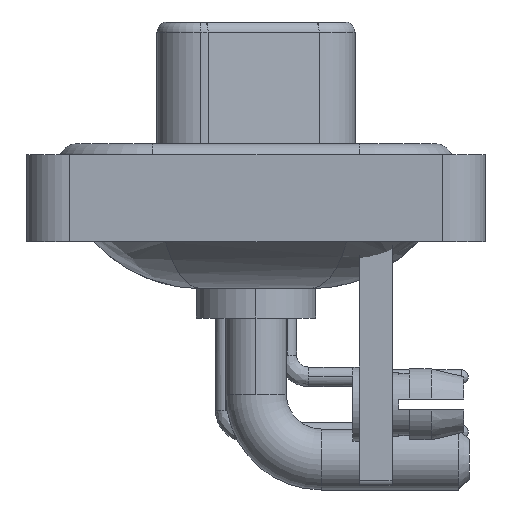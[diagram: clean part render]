
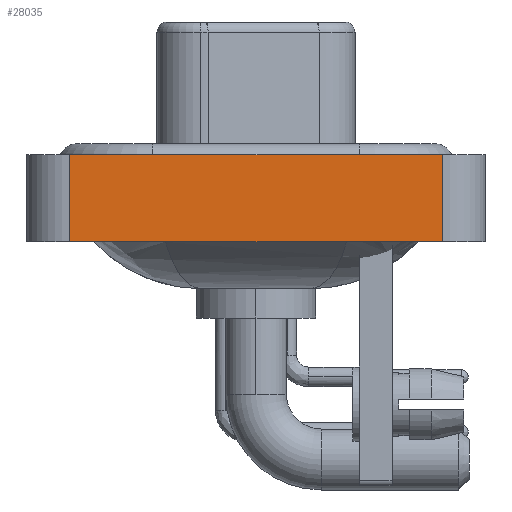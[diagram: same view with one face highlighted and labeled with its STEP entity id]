
A CAD part, left-side view. The second image highlights one B-rep face of the part: STEP entity #28035.
In plain terms, the highlighted planar face has unit normal (-1, 0, 0).
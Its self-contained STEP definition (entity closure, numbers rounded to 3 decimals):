
#370 = ORIENTED_EDGE ( 'NONE', *, *, #20379, .F. ) ;
#957 = PLANE ( 'NONE',  #3454 ) ;
#1491 = ORIENTED_EDGE ( 'NONE', *, *, #3482, .F. ) ;
#3369 = ORIENTED_EDGE ( 'NONE', *, *, #29128, .T. ) ;
#3454 = AXIS2_PLACEMENT_3D ( 'NONE', #12656, #7998, #15061 ) ;
#3482 = EDGE_CURVE ( 'NONE', #14479, #16802, #16844, .T. ) ;
#4682 = CARTESIAN_POINT ( 'NONE',  ( -7.35, -8.55, 0.4 ) ) ;
#5179 = LINE ( 'NONE', #8020, #21669 ) ;
#5720 = ORIENTED_EDGE ( 'NONE', *, *, #23602, .T. ) ;
#7998 = DIRECTION ( 'NONE',  ( -1., 0., 0. ) ) ;
#8020 = CARTESIAN_POINT ( 'NONE',  ( -7.35, -8.55, -3.6 ) ) ;
#8876 = CARTESIAN_POINT ( 'NONE',  ( -7.35, 8.55, 0.4 ) ) ;
#9983 = VECTOR ( 'NONE', #11663, 1000. ) ;
#11663 = DIRECTION ( 'NONE',  ( 0., 0., 1. ) ) ;
#12656 = CARTESIAN_POINT ( 'NONE',  ( -7.35, -8.55, -3.6 ) ) ;
#12820 = LINE ( 'NONE', #15232, #28074 ) ;
#14479 = VERTEX_POINT ( 'NONE', #8876 ) ;
#14735 = DIRECTION ( 'NONE',  ( 0., -1., 0. ) ) ;
#15061 = DIRECTION ( 'NONE',  ( 0., 0., 1. ) ) ;
#15232 = CARTESIAN_POINT ( 'NONE',  ( -7.35, 8.55, -3.6 ) ) ;
#15689 = VERTEX_POINT ( 'NONE', #28064 ) ;
#15882 = CARTESIAN_POINT ( 'NONE',  ( -7.35, -8.55, -3.6 ) ) ;
#16802 = VERTEX_POINT ( 'NONE', #4682 ) ;
#16844 = LINE ( 'NONE', #21613, #18081 ) ;
#17177 = DIRECTION ( 'NONE',  ( 0., -1., 0. ) ) ;
#18081 = VECTOR ( 'NONE', #14735, 1000. ) ;
#19241 = EDGE_LOOP ( 'NONE', ( #3369, #1491, #370, #5720 ) ) ;
#20379 = EDGE_CURVE ( 'NONE', #15689, #14479, #12820, .T. ) ;
#21613 = CARTESIAN_POINT ( 'NONE',  ( -7.35, -8.55, 0.4 ) ) ;
#21669 = VECTOR ( 'NONE', #17177, 1000. ) ;
#23602 = EDGE_CURVE ( 'NONE', #15689, #27837, #5179, .T. ) ;
#24408 = CARTESIAN_POINT ( 'NONE',  ( -7.35, -8.55, -3.6 ) ) ;
#25296 = LINE ( 'NONE', #15882, #9983 ) ;
#26754 = DIRECTION ( 'NONE',  ( 0., 0., 1. ) ) ;
#27837 = VERTEX_POINT ( 'NONE', #24408 ) ;
#28035 = ADVANCED_FACE ( 'NONE', ( #28683 ), #957, .T. ) ;
#28064 = CARTESIAN_POINT ( 'NONE',  ( -7.35, 8.55, -3.6 ) ) ;
#28074 = VECTOR ( 'NONE', #26754, 1000. ) ;
#28683 = FACE_OUTER_BOUND ( 'NONE', #19241, .T. ) ;
#29128 = EDGE_CURVE ( 'NONE', #27837, #16802, #25296, .T. ) ;
